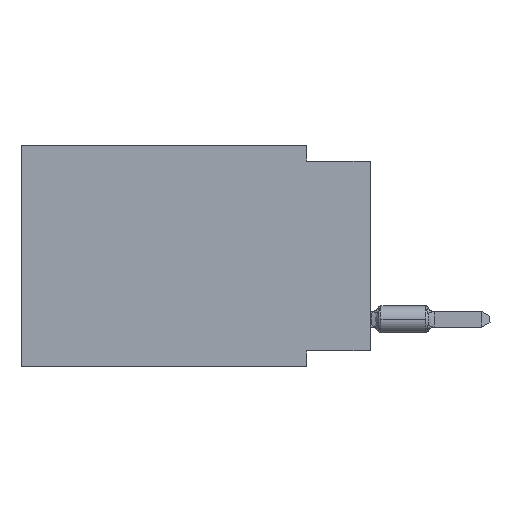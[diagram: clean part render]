
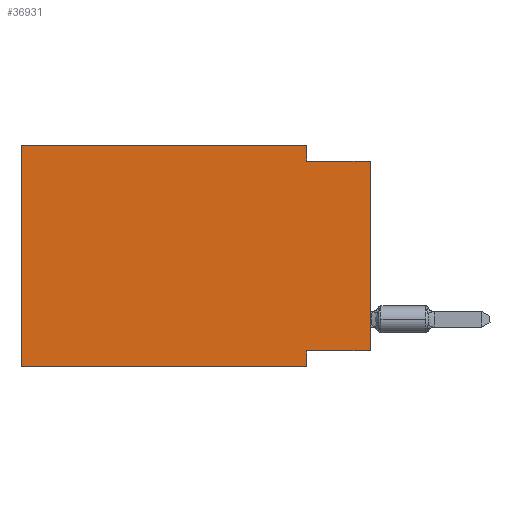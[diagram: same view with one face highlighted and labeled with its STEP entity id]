
A CAD part, left-side view. The second image highlights one B-rep face of the part: STEP entity #36931.
In plain terms, the highlighted planar face has unit normal (-1, 0, 0).
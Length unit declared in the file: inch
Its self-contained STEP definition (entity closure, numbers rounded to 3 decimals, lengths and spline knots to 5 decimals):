
#1840 = VECTOR ( 'NONE', #28580, 39.37008 ) ;
#2252 = ORIENTED_EDGE ( 'NONE', *, *, #31808, .T. ) ;
#2700 = CARTESIAN_POINT ( 'NONE',  ( 0., 0.55, 0. ) ) ;
#2923 = VECTOR ( 'NONE', #21397, 39.37008 ) ;
#4394 = LINE ( 'NONE', #13531, #35500 ) ;
#4445 = VERTEX_POINT ( 'NONE', #4987 ) ;
#4839 = CARTESIAN_POINT ( 'NONE',  ( 0., 0.55, 0. ) ) ;
#4987 = CARTESIAN_POINT ( 'NONE',  ( 0., 0.55, 0. ) ) ;
#6267 = VERTEX_POINT ( 'NONE', #36806 ) ;
#6858 = EDGE_CURVE ( 'NONE', #18053, #33470, #35853, .T. ) ;
#8556 = DIRECTION ( 'NONE',  ( 0., -1., 0. ) ) ;
#9320 = DIRECTION ( 'NONE',  ( 0., 0., -1. ) ) ;
#9676 = PLANE ( 'NONE',  #33074 ) ;
#9794 = CARTESIAN_POINT ( 'NONE',  ( 0., 0., -0.025 ) ) ;
#10066 = ORIENTED_EDGE ( 'NONE', *, *, #19896, .F. ) ;
#10165 = CARTESIAN_POINT ( 'NONE',  ( 0., 0.1, 0. ) ) ;
#10517 = DIRECTION ( 'NONE',  ( 0., 0., -1. ) ) ;
#10918 = VERTEX_POINT ( 'NONE', #20025 ) ;
#11750 = CARTESIAN_POINT ( 'NONE',  ( 0., 0.55, -0.35 ) ) ;
#12459 = LINE ( 'NONE', #11750, #2923 ) ;
#12984 = ORIENTED_EDGE ( 'NONE', *, *, #41067, .F. ) ;
#13531 = CARTESIAN_POINT ( 'NONE',  ( 0., 0., -0.325 ) ) ;
#14325 = VERTEX_POINT ( 'NONE', #40438 ) ;
#15577 = VECTOR ( 'NONE', #9320, 39.37008 ) ;
#15632 = VERTEX_POINT ( 'NONE', #23634 ) ;
#16380 = VECTOR ( 'NONE', #8556, 39.37008 ) ;
#16697 = DIRECTION ( 'NONE',  ( 0., 1., 0. ) ) ;
#17263 = DIRECTION ( 'NONE',  ( 0., -1., 0. ) ) ;
#17893 = EDGE_CURVE ( 'NONE', #10918, #25582, #40000, .T. ) ;
#18053 = VERTEX_POINT ( 'NONE', #32512 ) ;
#19015 = CARTESIAN_POINT ( 'NONE',  ( 0., 0.55, 0. ) ) ;
#19229 = VECTOR ( 'NONE', #17263, 39.37008 ) ;
#19896 = EDGE_CURVE ( 'NONE', #15632, #25582, #24899, .T. ) ;
#20025 = CARTESIAN_POINT ( 'NONE',  ( 0., 0., -0.325 ) ) ;
#20245 = VECTOR ( 'NONE', #10517, 39.37008 ) ;
#21397 = DIRECTION ( 'NONE',  ( 0., -1., 0. ) ) ;
#21518 = EDGE_CURVE ( 'NONE', #4445, #14325, #31823, .T. ) ;
#22716 = CARTESIAN_POINT ( 'NONE',  ( 0., 0., 0. ) ) ;
#23267 = CARTESIAN_POINT ( 'NONE',  ( 0., 0.1, -0.35 ) ) ;
#23634 = CARTESIAN_POINT ( 'NONE',  ( 0., 0.1, -0.025 ) ) ;
#24899 = LINE ( 'NONE', #30685, #16380 ) ;
#25582 = VERTEX_POINT ( 'NONE', #9794 ) ;
#25790 = ORIENTED_EDGE ( 'NONE', *, *, #6858, .F. ) ;
#26326 = EDGE_CURVE ( 'NONE', #10918, #18053, #4394, .T. ) ;
#26603 = ORIENTED_EDGE ( 'NONE', *, *, #26326, .F. ) ;
#27148 = CARTESIAN_POINT ( 'NONE',  ( 0., 0.1, -0.35 ) ) ;
#27538 = FACE_OUTER_BOUND ( 'NONE', #36813, .T. ) ;
#28565 = ORIENTED_EDGE ( 'NONE', *, *, #21518, .F. ) ;
#28580 = DIRECTION ( 'NONE',  ( 0., 0., 1. ) ) ;
#28912 = LINE ( 'NONE', #2700, #1840 ) ;
#29300 = ORIENTED_EDGE ( 'NONE', *, *, #17893, .T. ) ;
#30667 = LINE ( 'NONE', #10165, #15577 ) ;
#30685 = CARTESIAN_POINT ( 'NONE',  ( 0., 0., -0.025 ) ) ;
#30942 = VECTOR ( 'NONE', #41526, 39.37008 ) ;
#31808 = EDGE_CURVE ( 'NONE', #6267, #33470, #12459, .T. ) ;
#31823 = LINE ( 'NONE', #4839, #19229 ) ;
#32079 = DIRECTION ( 'NONE',  ( 0., 0., -1. ) ) ;
#32512 = CARTESIAN_POINT ( 'NONE',  ( 0., 0.1, -0.325 ) ) ;
#33033 = EDGE_CURVE ( 'NONE', #6267, #4445, #28912, .T. ) ;
#33074 = AXIS2_PLACEMENT_3D ( 'NONE', #19015, #38409, #32079 ) ;
#33470 = VERTEX_POINT ( 'NONE', #27148 ) ;
#35500 = VECTOR ( 'NONE', #16697, 39.37008 ) ;
#35812 = ORIENTED_EDGE ( 'NONE', *, *, #33033, .F. ) ;
#35853 = LINE ( 'NONE', #23267, #20245 ) ;
#36806 = CARTESIAN_POINT ( 'NONE',  ( 0., 0.55, -0.35 ) ) ;
#36813 = EDGE_LOOP ( 'NONE', ( #29300, #10066, #12984, #28565, #35812, #2252, #25790, #26603 ) ) ;
#36931 = ADVANCED_FACE ( 'NONE', ( #27538 ), #9676, .F. ) ;
#38409 = DIRECTION ( 'NONE',  ( 1., 0., 0. ) ) ;
#40000 = LINE ( 'NONE', #22716, #30942 ) ;
#40438 = CARTESIAN_POINT ( 'NONE',  ( 0., 0.1, 0. ) ) ;
#41067 = EDGE_CURVE ( 'NONE', #14325, #15632, #30667, .T. ) ;
#41526 = DIRECTION ( 'NONE',  ( 0., 0., 1. ) ) ;
